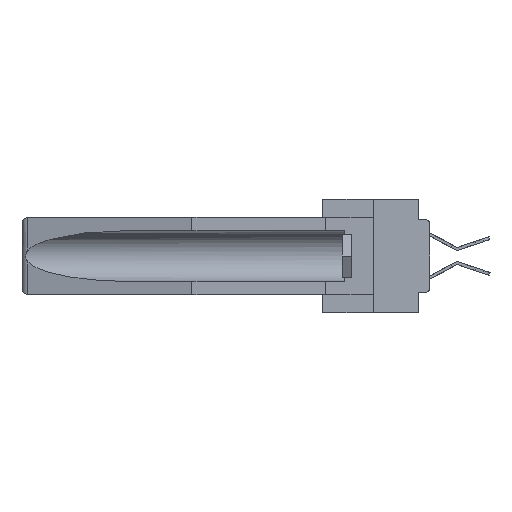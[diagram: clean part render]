
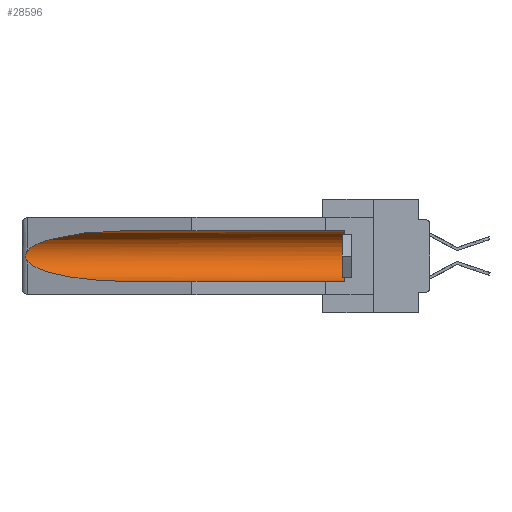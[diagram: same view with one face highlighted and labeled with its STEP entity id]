
A CAD part, left-side view. The second image highlights one B-rep face of the part: STEP entity #28596.
In plain terms, the highlighted cylindrical face has radius 2.857 mm (diameter 5.715 mm), a partial arc.
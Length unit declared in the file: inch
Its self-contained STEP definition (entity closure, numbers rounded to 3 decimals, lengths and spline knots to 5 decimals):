
#150 = CARTESIAN_POINT ( 'NONE',  ( 0.155, 1.07973, -0.059 ) ) ;
#328 = VERTEX_POINT ( 'NONE', #32611 ) ;
#450 = CARTESIAN_POINT ( 'NONE',  ( 0.155, -0.30754, -0.1715 ) ) ;
#671 = CARTESIAN_POINT ( 'NONE',  ( 0.155, 0.126, -0.1715 ) ) ;
#1270 = CARTESIAN_POINT ( 'NONE',  ( 0.26537, 1.52718, -0.19328 ) ) ;
#1397 = EDGE_CURVE ( 'NONE', #12506, #24469, #7074, .T. ) ;
#1428 = VECTOR ( 'NONE', #17319, 39.37008 ) ;
#1606 = CARTESIAN_POINT ( 'NONE',  ( 0.26537, 1.52718, -0.14972 ) ) ;
#1709 = CARTESIAN_POINT ( 'NONE',  ( 0.2673, 1.5327, -0.16383 ) ) ;
#1923 = VERTEX_POINT ( 'NONE', #14725 ) ;
#2140 = ORIENTED_EDGE ( 'NONE', *, *, #25850, .T. ) ;
#2482 = EDGE_CURVE ( 'NONE', #31302, #12506, #8552, .T. ) ;
#2588 = LINE ( 'NONE', #25068, #31268 ) ;
#3439 = EDGE_LOOP ( 'NONE', ( #12670, #25148, #13890, #17899, #17069, #2140 ) ) ;
#3564 =( BOUNDED_CURVE ( )  B_SPLINE_CURVE ( 3, ( #150, #18208, #18321, #23486 ),
 .UNSPECIFIED., .F., .F. ) 
 B_SPLINE_CURVE_WITH_KNOTS ( ( 4, 4 ),
 ( 4.71239, 6.08839 ),
 .UNSPECIFIED. ) 
 CURVE ( )  GEOMETRIC_REPRESENTATION_ITEM ( )  RATIONAL_B_SPLINE_CURVE ( ( 1., 0.848, 0.848, 1. ) ) 
 REPRESENTATION_ITEM ( '' )  );
#4206 = CARTESIAN_POINT ( 'NONE',  ( 0.26597, 1.52961, -0.15275 ) ) ;
#4313 = CARTESIAN_POINT ( 'NONE',  ( 0.2673, 1.53269, -0.17917 ) ) ;
#5182 = CARTESIAN_POINT ( 'NONE',  ( 0.26537, 1.52718, -0.19328 ) ) ;
#5547 = CYLINDRICAL_SURFACE ( 'NONE', #27479, 0.1125 ) ;
#6934 = CARTESIAN_POINT ( 'NONE',  ( 0.25451, 1.48313, -0.24835 ) ) ;
#7074 =( BOUNDED_CURVE ( )  B_SPLINE_CURVE ( 3, ( #17619, #6934, #9567, #32999 ),
 .UNSPECIFIED., .F., .F. ) 
 B_SPLINE_CURVE_WITH_KNOTS ( ( 4, 4 ),
 ( 0.1948, 1.5708 ),
 .UNSPECIFIED. ) 
 CURVE ( )  GEOMETRIC_REPRESENTATION_ITEM ( )  RATIONAL_B_SPLINE_CURVE ( ( 1., 0.848, 0.848, 1. ) ) 
 REPRESENTATION_ITEM ( '' )  );
#7895 = LINE ( 'NONE', #20018, #1428 ) ;
#8552 = B_SPLINE_CURVE_WITH_KNOTS ( 'NONE', 3,
 ( #1606, #4206, #26992, #1709, #11555, #19755, #4313, #29574, #32199, #1270 ),
 .UNSPECIFIED., .F., .F.,
 ( 4, 2, 2, 2, 4 ),
 ( 0., 0.00029, 0.00058, 0.00087, 0.00117 ),
 .UNSPECIFIED. ) ;
#8711 = DIRECTION ( 'NONE',  ( 0., -1., 0. ) ) ;
#9567 = CARTESIAN_POINT ( 'NONE',  ( 0.21114, 1.30732, -0.284 ) ) ;
#9953 = EDGE_CURVE ( 'NONE', #328, #1923, #32894, .T. ) ;
#11555 = CARTESIAN_POINT ( 'NONE',  ( 0.2675, 1.53308, -0.16763 ) ) ;
#12506 = VERTEX_POINT ( 'NONE', #5182 ) ;
#12670 = ORIENTED_EDGE ( 'NONE', *, *, #27961, .T. ) ;
#13890 = ORIENTED_EDGE ( 'NONE', *, *, #1397, .T. ) ;
#14725 = CARTESIAN_POINT ( 'NONE',  ( 0.155, 0.126, -0.059 ) ) ;
#15378 = CARTESIAN_POINT ( 'NONE',  ( 0.155, 1.07973, -0.284 ) ) ;
#15901 = DIRECTION ( 'NONE',  ( 0., 1., 0. ) ) ;
#16346 = DIRECTION ( 'NONE',  ( 0., 0., 1. ) ) ;
#16887 = VERTEX_POINT ( 'NONE', #31347 ) ;
#17069 = ORIENTED_EDGE ( 'NONE', *, *, #9953, .T. ) ;
#17319 = DIRECTION ( 'NONE',  ( 0., 1., 0. ) ) ;
#17619 = CARTESIAN_POINT ( 'NONE',  ( 0.26537, 1.52718, -0.19328 ) ) ;
#17899 = ORIENTED_EDGE ( 'NONE', *, *, #26444, .F. ) ;
#18208 = CARTESIAN_POINT ( 'NONE',  ( 0.21114, 1.30732, -0.059 ) ) ;
#18276 = DIRECTION ( 'NONE',  ( 0., 0., 1. ) ) ;
#18321 = CARTESIAN_POINT ( 'NONE',  ( 0.25451, 1.48313, -0.09465 ) ) ;
#19755 = CARTESIAN_POINT ( 'NONE',  ( 0.2675, 1.53308, -0.17534 ) ) ;
#20018 = CARTESIAN_POINT ( 'NONE',  ( 0.155, -0.30754, -0.059 ) ) ;
#23486 = CARTESIAN_POINT ( 'NONE',  ( 0.26537, 1.52718, -0.14972 ) ) ;
#24469 = VERTEX_POINT ( 'NONE', #15378 ) ;
#25068 = CARTESIAN_POINT ( 'NONE',  ( 0.155, -0.30754, -0.284 ) ) ;
#25148 = ORIENTED_EDGE ( 'NONE', *, *, #2482, .T. ) ;
#25850 = EDGE_CURVE ( 'NONE', #1923, #16887, #7895, .T. ) ;
#26444 = EDGE_CURVE ( 'NONE', #328, #24469, #2588, .T. ) ;
#26992 = CARTESIAN_POINT ( 'NONE',  ( 0.26654, 1.53092, -0.15636 ) ) ;
#27479 = AXIS2_PLACEMENT_3D ( 'NONE', #450, #15901, #18276 ) ;
#27961 = EDGE_CURVE ( 'NONE', #16887, #31302, #3564, .T. ) ;
#28205 = AXIS2_PLACEMENT_3D ( 'NONE', #671, #8711, #16346 ) ;
#28596 = ADVANCED_FACE ( 'NONE', ( #31383 ), #5547, .F. ) ;
#28849 = CARTESIAN_POINT ( 'NONE',  ( 0.26537, 1.52718, -0.14972 ) ) ;
#29574 = CARTESIAN_POINT ( 'NONE',  ( 0.26655, 1.53094, -0.18657 ) ) ;
#30269 = DIRECTION ( 'NONE',  ( 0., 1., 0. ) ) ;
#31268 = VECTOR ( 'NONE', #30269, 39.37008 ) ;
#31302 = VERTEX_POINT ( 'NONE', #28849 ) ;
#31347 = CARTESIAN_POINT ( 'NONE',  ( 0.155, 1.07973, -0.059 ) ) ;
#31383 = FACE_OUTER_BOUND ( 'NONE', #3439, .T. ) ;
#32199 = CARTESIAN_POINT ( 'NONE',  ( 0.26597, 1.5296, -0.19026 ) ) ;
#32611 = CARTESIAN_POINT ( 'NONE',  ( 0.155, 0.126, -0.284 ) ) ;
#32894 = CIRCLE ( 'NONE', #28205, 0.1125 ) ;
#32999 = CARTESIAN_POINT ( 'NONE',  ( 0.155, 1.07973, -0.284 ) ) ;
